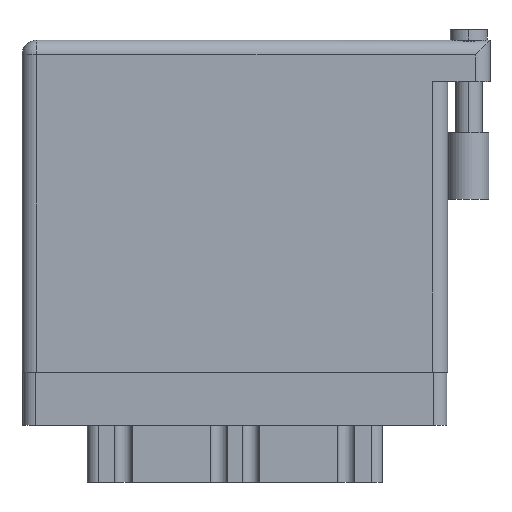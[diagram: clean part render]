
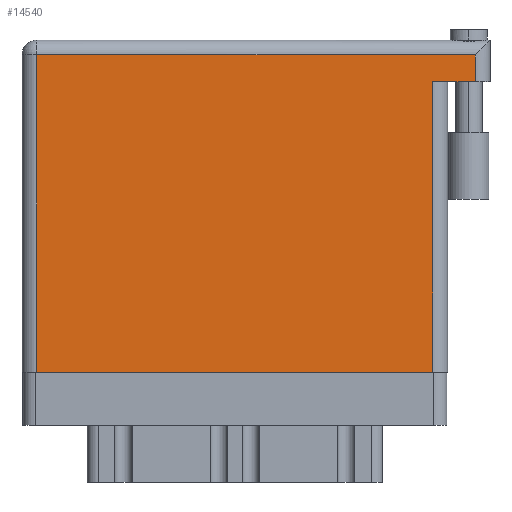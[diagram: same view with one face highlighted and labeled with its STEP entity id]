
A CAD part, front view. The second image highlights one B-rep face of the part: STEP entity #14540.
In plain terms, the highlighted face is planar.
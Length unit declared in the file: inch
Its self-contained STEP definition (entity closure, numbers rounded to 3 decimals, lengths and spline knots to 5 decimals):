
#640 = CARTESIAN_POINT ( 'NONE',  ( 0., 1.496, 0. ) ) ;
#1355 = LINE ( 'NONE', #19229, #21860 ) ;
#2632 = VECTOR ( 'NONE', #35597, 39.37008 ) ;
#3627 = DIRECTION ( 'NONE',  ( 0., 0., -1. ) ) ;
#6845 = CARTESIAN_POINT ( 'NONE',  ( 2.208, 1.369, 0. ) ) ;
#8392 = VERTEX_POINT ( 'NONE', #15151 ) ;
#8481 = VECTOR ( 'NONE', #31874, 39.37008 ) ;
#8661 = ORIENTED_EDGE ( 'NONE', *, *, #25342, .T. ) ;
#9509 = DIRECTION ( 'NONE',  ( 1., 0., 0. ) ) ;
#10031 = DIRECTION ( 'NONE',  ( 0., 1., 0. ) ) ;
#10076 = CARTESIAN_POINT ( 'NONE',  ( 0.07, 1.496, 0. ) ) ;
#12182 = CARTESIAN_POINT ( 'NONE',  ( 1.938, 1.369, 0. ) ) ;
#12353 = FACE_OUTER_BOUND ( 'NONE', #32437, .T. ) ;
#12424 = VERTEX_POINT ( 'NONE', #24216 ) ;
#13637 = ORIENTED_EDGE ( 'NONE', *, *, #26130, .T. ) ;
#14397 = VECTOR ( 'NONE', #10031, 39.37008 ) ;
#14476 = CARTESIAN_POINT ( 'NONE',  ( 2.138, 1.496, 0. ) ) ;
#14540 = ADVANCED_FACE ( 'NONE', ( #12353 ), #24231, .F. ) ;
#15151 = CARTESIAN_POINT ( 'NONE',  ( 1.938, 0., 0. ) ) ;
#16005 = LINE ( 'NONE', #6845, #8481 ) ;
#16092 = CARTESIAN_POINT ( 'NONE',  ( 0.07, 0., 0. ) ) ;
#17149 = VECTOR ( 'NONE', #24350, 39.37008 ) ;
#18006 = AXIS2_PLACEMENT_3D ( 'NONE', #35344, #3627, #21305 ) ;
#18133 = LINE ( 'NONE', #640, #17149 ) ;
#19229 = CARTESIAN_POINT ( 'NONE',  ( 2.138, 1.566, 0. ) ) ;
#19347 = VERTEX_POINT ( 'NONE', #16092 ) ;
#21163 = LINE ( 'NONE', #26262, #2632 ) ;
#21305 = DIRECTION ( 'NONE',  ( -1., 0., 0. ) ) ;
#21860 = VECTOR ( 'NONE', #30907, 39.37008 ) ;
#22553 = ORIENTED_EDGE ( 'NONE', *, *, #36862, .F. ) ;
#23399 = VECTOR ( 'NONE', #9509, 39.37008 ) ;
#24216 = CARTESIAN_POINT ( 'NONE',  ( 2.138, 1.369, 0. ) ) ;
#24231 = PLANE ( 'NONE',  #18006 ) ;
#24350 = DIRECTION ( 'NONE',  ( -1., 0., 0. ) ) ;
#24402 = VERTEX_POINT ( 'NONE', #24641 ) ;
#24641 = CARTESIAN_POINT ( 'NONE',  ( 1.938, 1.369, 0. ) ) ;
#24821 = LINE ( 'NONE', #12182, #14397 ) ;
#25342 = EDGE_CURVE ( 'NONE', #8392, #24402, #24821, .T. ) ;
#26130 = EDGE_CURVE ( 'NONE', #33342, #19347, #21163, .T. ) ;
#26262 = CARTESIAN_POINT ( 'NONE',  ( 0.07, 0., 0. ) ) ;
#26406 = ORIENTED_EDGE ( 'NONE', *, *, #28760, .T. ) ;
#26844 = LINE ( 'NONE', #30140, #23399 ) ;
#27317 = EDGE_CURVE ( 'NONE', #12424, #34171, #1355, .T. ) ;
#28760 = EDGE_CURVE ( 'NONE', #34171, #33342, #18133, .T. ) ;
#29104 = EDGE_CURVE ( 'NONE', #19347, #8392, #26844, .T. ) ;
#30140 = CARTESIAN_POINT ( 'NONE',  ( 0., 0., 0. ) ) ;
#30907 = DIRECTION ( 'NONE',  ( 0., 1., 0. ) ) ;
#31874 = DIRECTION ( 'NONE',  ( -1., 0., 0. ) ) ;
#32437 = EDGE_LOOP ( 'NONE', ( #33909, #8661, #22553, #34614, #26406, #13637 ) ) ;
#33342 = VERTEX_POINT ( 'NONE', #10076 ) ;
#33909 = ORIENTED_EDGE ( 'NONE', *, *, #29104, .T. ) ;
#34171 = VERTEX_POINT ( 'NONE', #14476 ) ;
#34614 = ORIENTED_EDGE ( 'NONE', *, *, #27317, .T. ) ;
#35344 = CARTESIAN_POINT ( 'NONE',  ( 0., 1.566, 0. ) ) ;
#35597 = DIRECTION ( 'NONE',  ( 0., -1., 0. ) ) ;
#36862 = EDGE_CURVE ( 'NONE', #12424, #24402, #16005, .T. ) ;
